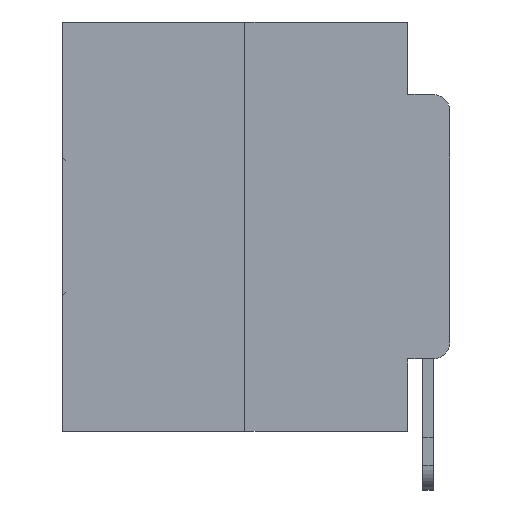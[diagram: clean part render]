
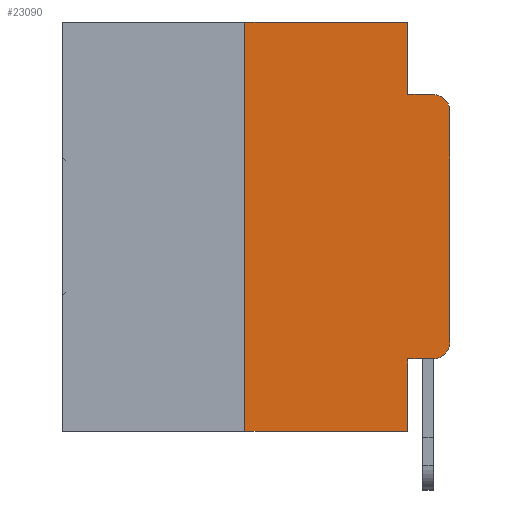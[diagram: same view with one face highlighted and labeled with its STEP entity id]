
A CAD part, left-side view. The second image highlights one B-rep face of the part: STEP entity #23090.
In plain terms, the highlighted planar face has unit normal (-1, 0, 0).
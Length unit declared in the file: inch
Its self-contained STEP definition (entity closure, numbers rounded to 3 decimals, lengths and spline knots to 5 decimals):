
#3 = FACE_OUTER_BOUND ( 'NONE', #26681, .T. ) ;
#199 = DIRECTION ( 'NONE',  ( 0., 0., -1. ) ) ;
#334 = VECTOR ( 'NONE', #199, 39.37008 ) ;
#2099 = AXIS2_PLACEMENT_3D ( 'NONE', #31894, #2449, #19803 ) ;
#2449 = DIRECTION ( 'NONE',  ( 1., 0., 0. ) ) ;
#2486 = DIRECTION ( 'NONE',  ( 0., 0., -1. ) ) ;
#2513 = VERTEX_POINT ( 'NONE', #23504 ) ;
#2637 = EDGE_CURVE ( 'NONE', #2513, #19542, #10586, .T. ) ;
#2910 = LINE ( 'NONE', #27251, #21860 ) ;
#3691 = EDGE_CURVE ( 'NONE', #28776, #3996, #13946, .T. ) ;
#3996 = VERTEX_POINT ( 'NONE', #7515 ) ;
#4430 = EDGE_CURVE ( 'NONE', #5461, #6921, #26432, .T. ) ;
#4476 = EDGE_CURVE ( 'NONE', #6921, #14504, #25646, .T. ) ;
#4482 = EDGE_CURVE ( 'NONE', #22082, #14504, #5439, .T. ) ;
#4492 = EDGE_CURVE ( 'NONE', #19542, #22082, #11937, .T. ) ;
#4530 = EDGE_CURVE ( 'NONE', #28776, #2513, #2910, .T. ) ;
#4584 = EDGE_CURVE ( 'NONE', #23873, #3996, #8132, .T. ) ;
#4588 = EDGE_CURVE ( 'NONE', #23873, #14907, #26033, .T. ) ;
#4683 = EDGE_CURVE ( 'NONE', #14907, #5461, #10020, .T. ) ;
#4739 = CARTESIAN_POINT ( 'NONE',  ( 0., 0.02, -0.4115 ) ) ;
#4766 = DIRECTION ( 'NONE',  ( 0., 0., 1. ) ) ;
#5092 = CARTESIAN_POINT ( 'NONE',  ( 0., 0.02, -0.1085 ) ) ;
#5439 = LINE ( 'NONE', #19728, #30573 ) ;
#5461 = VERTEX_POINT ( 'NONE', #26298 ) ;
#5935 = ORIENTED_EDGE ( 'NONE', *, *, #4492, .F. ) ;
#6578 = VECTOR ( 'NONE', #15906, 39.37008 ) ;
#6921 = VERTEX_POINT ( 'NONE', #21959 ) ;
#7515 = CARTESIAN_POINT ( 'NONE',  ( 0., 0.051, -0.5 ) ) ;
#7576 = DIRECTION ( 'NONE',  ( 0., 0., -1. ) ) ;
#8132 = LINE ( 'NONE', #20255, #334 ) ;
#8223 = CARTESIAN_POINT ( 'NONE',  ( 0., 0.02, -0.0885 ) ) ;
#10020 = CIRCLE ( 'NONE', #16796, 0.02 ) ;
#10586 = LINE ( 'NONE', #31327, #22803 ) ;
#11867 = DIRECTION ( 'NONE',  ( 0., -1., 0. ) ) ;
#11937 = LINE ( 'NONE', #12466, #23376 ) ;
#12466 = CARTESIAN_POINT ( 'NONE',  ( 0., 0.051, 0. ) ) ;
#13427 = CARTESIAN_POINT ( 'NONE',  ( 0., 0.051, -0.4115 ) ) ;
#13460 = ORIENTED_EDGE ( 'NONE', *, *, #4430, .T. ) ;
#13866 = DIRECTION ( 'NONE',  ( -1., 0., 0. ) ) ;
#13946 = LINE ( 'NONE', #20753, #15491 ) ;
#14504 = VERTEX_POINT ( 'NONE', #8223 ) ;
#14907 = VERTEX_POINT ( 'NONE', #4739 ) ;
#14912 = PLANE ( 'NONE',  #2099 ) ;
#15170 = DIRECTION ( 'NONE',  ( 0., 0., 1. ) ) ;
#15491 = VECTOR ( 'NONE', #18294, 39.37008 ) ;
#15906 = DIRECTION ( 'NONE',  ( 0., -1., 0. ) ) ;
#16796 = AXIS2_PLACEMENT_3D ( 'NONE', #28429, #13866, #30842 ) ;
#17298 = DIRECTION ( 'NONE',  ( 0., -1., 0. ) ) ;
#18059 = ORIENTED_EDGE ( 'NONE', *, *, #3691, .T. ) ;
#18143 = CARTESIAN_POINT ( 'NONE',  ( 0., 0.051, -0.0885 ) ) ;
#18294 = DIRECTION ( 'NONE',  ( 0., -1., 0. ) ) ;
#19419 = CARTESIAN_POINT ( 'NONE',  ( 0., 0., 0. ) ) ;
#19542 = VERTEX_POINT ( 'NONE', #23419 ) ;
#19728 = CARTESIAN_POINT ( 'NONE',  ( 0., 0.051, -0.0885 ) ) ;
#19803 = DIRECTION ( 'NONE',  ( 0., 0., -1. ) ) ;
#19961 = VECTOR ( 'NONE', #4766, 39.37008 ) ;
#20255 = CARTESIAN_POINT ( 'NONE',  ( 0., 0.051, 0. ) ) ;
#20313 = CARTESIAN_POINT ( 'NONE',  ( 0., 0.25, -0.5 ) ) ;
#20753 = CARTESIAN_POINT ( 'NONE',  ( 0., 0.473, -0.5 ) ) ;
#21268 = ORIENTED_EDGE ( 'NONE', *, *, #2637, .F. ) ;
#21860 = VECTOR ( 'NONE', #15170, 39.37008 ) ;
#21959 = CARTESIAN_POINT ( 'NONE',  ( 0., 0., -0.1085 ) ) ;
#22082 = VERTEX_POINT ( 'NONE', #18143 ) ;
#22176 = DIRECTION ( 'NONE',  ( -1., 0., 0. ) ) ;
#22803 = VECTOR ( 'NONE', #11867, 39.37008 ) ;
#23090 = ADVANCED_FACE ( 'NONE', ( #3 ), #14912, .F. ) ;
#23336 = ORIENTED_EDGE ( 'NONE', *, *, #4530, .F. ) ;
#23376 = VECTOR ( 'NONE', #2486, 39.37008 ) ;
#23419 = CARTESIAN_POINT ( 'NONE',  ( 0., 0.051, 0. ) ) ;
#23504 = CARTESIAN_POINT ( 'NONE',  ( 0., 0.25, 0. ) ) ;
#23873 = VERTEX_POINT ( 'NONE', #25019 ) ;
#24509 = ORIENTED_EDGE ( 'NONE', *, *, #4683, .T. ) ;
#25019 = CARTESIAN_POINT ( 'NONE',  ( 0., 0.051, -0.4115 ) ) ;
#25308 = ORIENTED_EDGE ( 'NONE', *, *, #4482, .F. ) ;
#25509 = AXIS2_PLACEMENT_3D ( 'NONE', #5092, #22176, #7576 ) ;
#25646 = CIRCLE ( 'NONE', #25509, 0.02 ) ;
#26033 = LINE ( 'NONE', #13427, #6578 ) ;
#26298 = CARTESIAN_POINT ( 'NONE',  ( 0., 0., -0.3915 ) ) ;
#26432 = LINE ( 'NONE', #19419, #19961 ) ;
#26681 = EDGE_LOOP ( 'NONE', ( #13460, #28007, #25308, #5935, #21268, #23336, #18059, #26850, #28809, #24509 ) ) ;
#26850 = ORIENTED_EDGE ( 'NONE', *, *, #4584, .F. ) ;
#27251 = CARTESIAN_POINT ( 'NONE',  ( 0., 0.25, 0. ) ) ;
#28007 = ORIENTED_EDGE ( 'NONE', *, *, #4476, .T. ) ;
#28429 = CARTESIAN_POINT ( 'NONE',  ( 0., 0.02, -0.3915 ) ) ;
#28776 = VERTEX_POINT ( 'NONE', #20313 ) ;
#28809 = ORIENTED_EDGE ( 'NONE', *, *, #4588, .T. ) ;
#30573 = VECTOR ( 'NONE', #17298, 39.37008 ) ;
#30842 = DIRECTION ( 'NONE',  ( 0., 0., -1. ) ) ;
#31327 = CARTESIAN_POINT ( 'NONE',  ( 0., 0.473, 0. ) ) ;
#31894 = CARTESIAN_POINT ( 'NONE',  ( 0., 0.473, 0. ) ) ;
